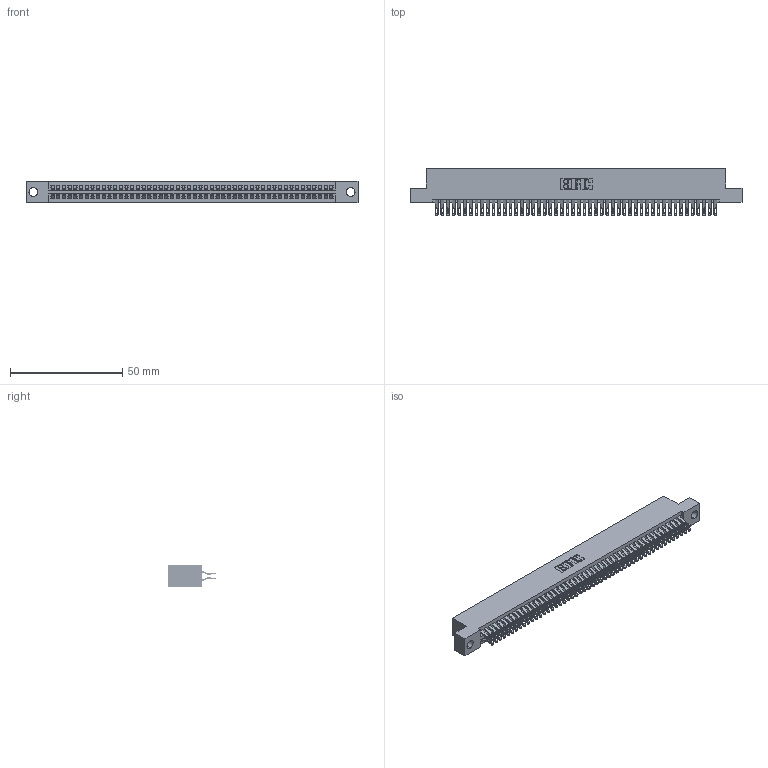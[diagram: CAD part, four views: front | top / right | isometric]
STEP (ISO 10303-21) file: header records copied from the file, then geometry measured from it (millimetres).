
FILE_DESCRIPTION (( 'STEP AP203' ), '1' );
FILE_NAME ('395-100-555-204.STEP', '2018-11-30T02:47:59', ( '' ), ( '' ), 'SwSTEP 2.0', 'SolidWorks 2016', '' );
FILE_SCHEMA (( 'CONFIG_CONTROL_DESIGN' ));
Length unit declared in the file: inch
Products named in the file (3): 395-100-555-204; 345-292-001_555 Tail; 345 Part_Flush Mounting Lugs - 0.156 Dia-TH
Assembly tree (101 placements, depth 2):
  395-100-555-204
    345 Part_Flush Mounting Lugs - 0.156 Dia-TH
    345-292-001_555 Tail  x100
Bounding box: 148.21 x 21.13 x 9.4 mm (x, y, z)
Volume: 14673.6 mm3; surface area: 22669.1 mm2
Topology: 101 solids, 101 shells, 5726 faces, 18041 edges, 12026 vertices
Faces by surface type: plane 3180, cylinder 2546
Entity records: 38483 total; most frequent: CARTESIAN_POINT 6478, ORIENTED_EDGE 6382, DIRECTION 5671, EDGE_CURVE 3191, LINE 2839, VECTOR 2839, VERTEX_POINT 2126, AXIS2_PLACEMENT_3D 1416
